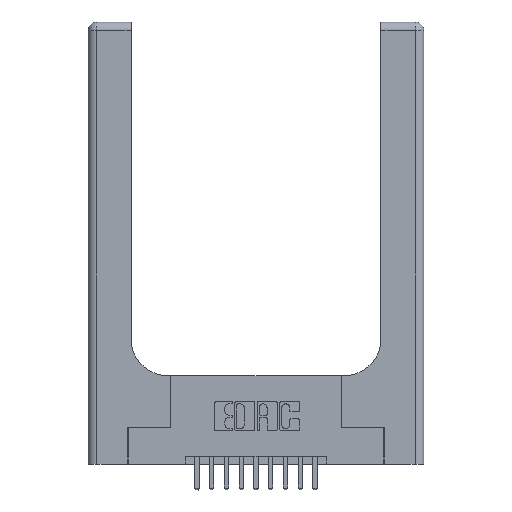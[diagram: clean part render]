
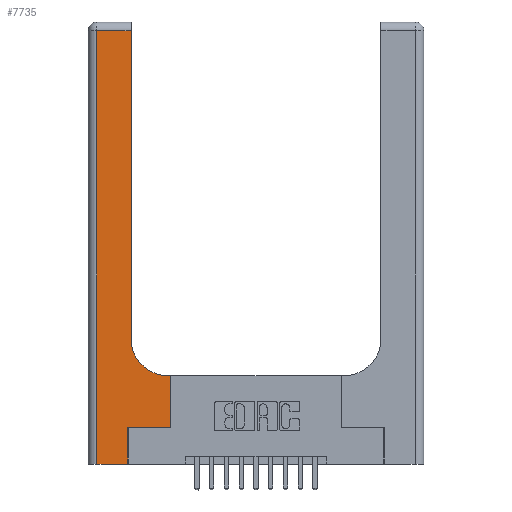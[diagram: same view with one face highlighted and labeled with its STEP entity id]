
A CAD part, top view. The second image highlights one B-rep face of the part: STEP entity #7735.
In plain terms, the highlighted planar face has unit normal (0, 0, 1).
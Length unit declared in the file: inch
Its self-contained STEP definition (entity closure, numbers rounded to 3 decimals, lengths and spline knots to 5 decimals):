
#319 = PLANE ( 'NONE',  #16535 ) ;
#628 = EDGE_CURVE ( 'NONE', #13061, #1603, #8227, .T. ) ;
#735 = DIRECTION ( 'NONE',  ( 0., -1., 0. ) ) ;
#1386 = DIRECTION ( 'NONE',  ( 0., 1., 0. ) ) ;
#1480 = ORIENTED_EDGE ( 'NONE', *, *, #10926, .T. ) ;
#1603 = VERTEX_POINT ( 'NONE', #14431 ) ;
#1627 = DIRECTION ( 'NONE',  ( 0., 0., -1. ) ) ;
#2223 = VECTOR ( 'NONE', #6169, 39.37008 ) ;
#2744 = AXIS2_PLACEMENT_3D ( 'NONE', #11367, #3622, #12657 ) ;
#2855 = FACE_OUTER_BOUND ( 'NONE', #3132, .T. ) ;
#3005 = VERTEX_POINT ( 'NONE', #3580 ) ;
#3132 = EDGE_LOOP ( 'NONE', ( #10205, #7381, #14177, #4793, #8465, #13245, #1480, #8300, #16106 ) ) ;
#3580 = CARTESIAN_POINT ( 'NONE',  ( 0.06, 2.94, 0.37 ) ) ;
#3622 = DIRECTION ( 'NONE',  ( 0., 0., -1. ) ) ;
#3655 = VECTOR ( 'NONE', #1386, 39.37008 ) ;
#3783 = EDGE_CURVE ( 'NONE', #14984, #13061, #6115, .T. ) ;
#3788 = EDGE_CURVE ( 'NONE', #13541, #8632, #12160, .T. ) ;
#3960 = VECTOR ( 'NONE', #14578, 39.37008 ) ;
#4525 = LINE ( 'NONE', #5765, #13193 ) ;
#4558 = EDGE_CURVE ( 'NONE', #8632, #9605, #4684, .T. ) ;
#4684 = LINE ( 'NONE', #9189, #3655 ) ;
#4793 = ORIENTED_EDGE ( 'NONE', *, *, #3783, .T. ) ;
#4815 = DIRECTION ( 'NONE',  ( 0., 1., 0. ) ) ;
#5765 = CARTESIAN_POINT ( 'NONE',  ( 0., 2.94, 0.37 ) ) ;
#6115 = LINE ( 'NONE', #15192, #2223 ) ;
#6135 = CARTESIAN_POINT ( 'NONE',  ( 0.2915, 0.85, 0.37 ) ) ;
#6169 = DIRECTION ( 'NONE',  ( 1., 0., 0. ) ) ;
#6315 = DIRECTION ( 'NONE',  ( 0., 1., 0. ) ) ;
#6779 = CARTESIAN_POINT ( 'NONE',  ( 0.269, 0.25, 0.37 ) ) ;
#6893 = VECTOR ( 'NONE', #12098, 39.37008 ) ;
#7019 = DIRECTION ( 'NONE',  ( -1., 0., 0. ) ) ;
#7380 = LINE ( 'NONE', #6779, #3960 ) ;
#7381 = ORIENTED_EDGE ( 'NONE', *, *, #8408, .T. ) ;
#7513 = VERTEX_POINT ( 'NONE', #12781 ) ;
#7735 = ADVANCED_FACE ( 'NONE', ( #2855 ), #319, .F. ) ;
#7812 = VECTOR ( 'NONE', #6315, 39.37008 ) ;
#7955 = CARTESIAN_POINT ( 'NONE',  ( 0.06, 0., 0.37 ) ) ;
#8227 = LINE ( 'NONE', #16345, #7812 ) ;
#8300 = ORIENTED_EDGE ( 'NONE', *, *, #9089, .T. ) ;
#8408 = EDGE_CURVE ( 'NONE', #9605, #3005, #4525, .T. ) ;
#8465 = ORIENTED_EDGE ( 'NONE', *, *, #628, .T. ) ;
#8632 = VERTEX_POINT ( 'NONE', #6135 ) ;
#8860 = VECTOR ( 'NONE', #4815, 39.37008 ) ;
#9089 = EDGE_CURVE ( 'NONE', #10744, #13541, #14171, .T. ) ;
#9189 = CARTESIAN_POINT ( 'NONE',  ( 0.2915, 3., 0.37 ) ) ;
#9538 = CARTESIAN_POINT ( 'NONE',  ( 0.269, 0., 0.37 ) ) ;
#9605 = VERTEX_POINT ( 'NONE', #11970 ) ;
#9634 = VECTOR ( 'NONE', #735, 39.37008 ) ;
#10205 = ORIENTED_EDGE ( 'NONE', *, *, #4558, .T. ) ;
#10743 = DIRECTION ( 'NONE',  ( -1., 0., 0. ) ) ;
#10744 = VERTEX_POINT ( 'NONE', #13293 ) ;
#10926 = EDGE_CURVE ( 'NONE', #7513, #10744, #11896, .T. ) ;
#11303 = CARTESIAN_POINT ( 'NONE',  ( 0.5585, 0.25, 0.37 ) ) ;
#11367 = CARTESIAN_POINT ( 'NONE',  ( 0.5415, 0.85, 0.37 ) ) ;
#11896 = LINE ( 'NONE', #11303, #8860 ) ;
#11970 = CARTESIAN_POINT ( 'NONE',  ( 0.2915, 2.94, 0.37 ) ) ;
#12001 = EDGE_CURVE ( 'NONE', #3005, #14984, #13064, .T. ) ;
#12098 = DIRECTION ( 'NONE',  ( -1., 0., 0. ) ) ;
#12160 = CIRCLE ( 'NONE', #2744, 0.25 ) ;
#12483 = EDGE_CURVE ( 'NONE', #1603, #7513, #7380, .T. ) ;
#12657 = DIRECTION ( 'NONE',  ( 1., 0., 0. ) ) ;
#12781 = CARTESIAN_POINT ( 'NONE',  ( 0.5585, 0.25, 0.37 ) ) ;
#13061 = VERTEX_POINT ( 'NONE', #9538 ) ;
#13064 = LINE ( 'NONE', #13688, #9634 ) ;
#13193 = VECTOR ( 'NONE', #7019, 39.37008 ) ;
#13245 = ORIENTED_EDGE ( 'NONE', *, *, #12483, .T. ) ;
#13284 = CARTESIAN_POINT ( 'NONE',  ( 0., 3., 0.37 ) ) ;
#13293 = CARTESIAN_POINT ( 'NONE',  ( 0.5585, 0.6, 0.37 ) ) ;
#13399 = CARTESIAN_POINT ( 'NONE',  ( 0.2915, 0.6, 0.37 ) ) ;
#13541 = VERTEX_POINT ( 'NONE', #14735 ) ;
#13688 = CARTESIAN_POINT ( 'NONE',  ( 0.06, 3., 0.37 ) ) ;
#14171 = LINE ( 'NONE', #13399, #6893 ) ;
#14177 = ORIENTED_EDGE ( 'NONE', *, *, #12001, .T. ) ;
#14431 = CARTESIAN_POINT ( 'NONE',  ( 0.269, 0.25, 0.37 ) ) ;
#14578 = DIRECTION ( 'NONE',  ( 1., 0., 0. ) ) ;
#14735 = CARTESIAN_POINT ( 'NONE',  ( 0.5415, 0.6, 0.37 ) ) ;
#14984 = VERTEX_POINT ( 'NONE', #7955 ) ;
#15192 = CARTESIAN_POINT ( 'NONE',  ( 0., 0., 0.37 ) ) ;
#16106 = ORIENTED_EDGE ( 'NONE', *, *, #3788, .T. ) ;
#16345 = CARTESIAN_POINT ( 'NONE',  ( 0.269, 0., 0.37 ) ) ;
#16535 = AXIS2_PLACEMENT_3D ( 'NONE', #13284, #1627, #10743 ) ;
